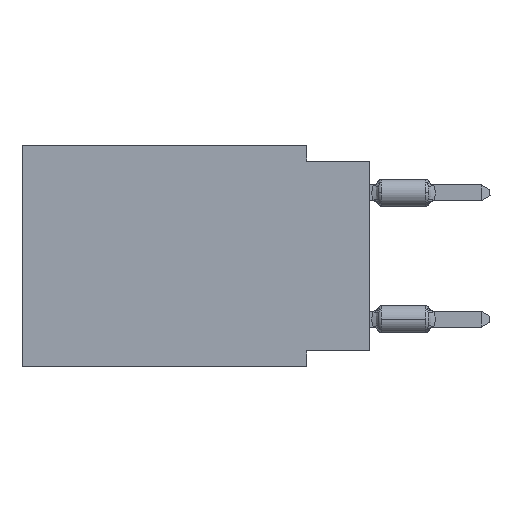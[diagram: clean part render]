
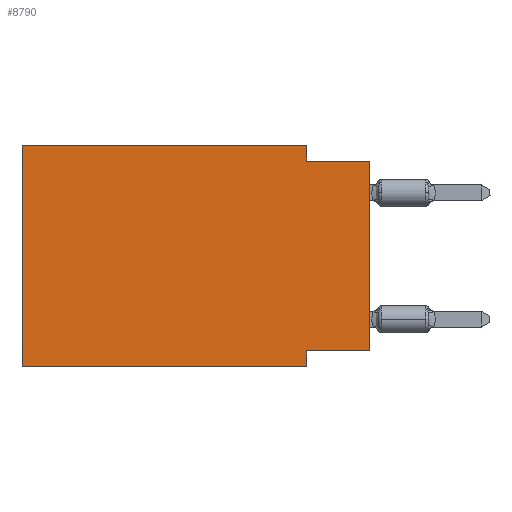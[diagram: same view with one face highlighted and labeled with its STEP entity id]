
A CAD part, left-side view. The second image highlights one B-rep face of the part: STEP entity #8790.
In plain terms, the highlighted planar face has unit normal (-1, 0, 0).
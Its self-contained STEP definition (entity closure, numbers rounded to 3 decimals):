
#327 = AXIS2_PLACEMENT_3D ( 'NONE', #10532, #20254, #37382 ) ;
#1716 = CARTESIAN_POINT ( 'NONE',  ( 0., 2.54, -8.89 ) ) ;
#2028 = VERTEX_POINT ( 'NONE', #53183 ) ;
#2197 = LINE ( 'NONE', #20183, #47291 ) ;
#2271 = PLANE ( 'NONE',  #327 ) ;
#3579 = CARTESIAN_POINT ( 'NONE',  ( 0., 13.97, 0. ) ) ;
#5478 = LINE ( 'NONE', #28453, #56012 ) ;
#7317 = CARTESIAN_POINT ( 'NONE',  ( 0., 2.54, 0. ) ) ;
#8790 = ADVANCED_FACE ( 'NONE', ( #19667 ), #2271, .F. ) ;
#9398 = VECTOR ( 'NONE', #21600, 1000. ) ;
#10532 = CARTESIAN_POINT ( 'NONE',  ( 0., 13.97, 0. ) ) ;
#11060 = DIRECTION ( 'NONE',  ( 0., -1., 0. ) ) ;
#11379 = DIRECTION ( 'NONE',  ( 0., 0., 1. ) ) ;
#12383 = VECTOR ( 'NONE', #16252, 1000. ) ;
#12592 = ORIENTED_EDGE ( 'NONE', *, *, #21545, .F. ) ;
#12681 = VECTOR ( 'NONE', #56651, 1000. ) ;
#12955 = VECTOR ( 'NONE', #26586, 1000. ) ;
#13992 = VERTEX_POINT ( 'NONE', #37721 ) ;
#14614 = VECTOR ( 'NONE', #56558, 1000. ) ;
#14849 = EDGE_CURVE ( 'NONE', #48085, #39375, #24808, .T. ) ;
#15495 = DIRECTION ( 'NONE',  ( 0., 0., -1. ) ) ;
#16252 = DIRECTION ( 'NONE',  ( 0., 0., 1. ) ) ;
#16602 = ORIENTED_EDGE ( 'NONE', *, *, #47740, .F. ) ;
#17611 = ORIENTED_EDGE ( 'NONE', *, *, #43153, .T. ) ;
#19488 = CARTESIAN_POINT ( 'NONE',  ( 0., 13.97, 0. ) ) ;
#19639 = CARTESIAN_POINT ( 'NONE',  ( 0., 0., 0. ) ) ;
#19667 = FACE_OUTER_BOUND ( 'NONE', #22935, .T. ) ;
#20183 = CARTESIAN_POINT ( 'NONE',  ( 0., 13.97, -8.89 ) ) ;
#20254 = DIRECTION ( 'NONE',  ( 1., 0., 0. ) ) ;
#20385 = CARTESIAN_POINT ( 'NONE',  ( 0., 0., -0.635 ) ) ;
#21545 = EDGE_CURVE ( 'NONE', #54140, #41581, #52586, .T. ) ;
#21600 = DIRECTION ( 'NONE',  ( 0., 1., 0. ) ) ;
#22935 = EDGE_LOOP ( 'NONE', ( #57510, #30529, #39712, #31897, #30223, #17611, #16602, #12592 ) ) ;
#24808 = LINE ( 'NONE', #20385, #12681 ) ;
#25574 = LINE ( 'NONE', #7317, #14614 ) ;
#25982 = LINE ( 'NONE', #3579, #12383 ) ;
#26586 = DIRECTION ( 'NONE',  ( 0., -1., 0. ) ) ;
#26988 = VERTEX_POINT ( 'NONE', #1716 ) ;
#28302 = VERTEX_POINT ( 'NONE', #19488 ) ;
#28453 = CARTESIAN_POINT ( 'NONE',  ( 0., 2.54, -8.89 ) ) ;
#30223 = ORIENTED_EDGE ( 'NONE', *, *, #42631, .F. ) ;
#30529 = ORIENTED_EDGE ( 'NONE', *, *, #14849, .F. ) ;
#31897 = ORIENTED_EDGE ( 'NONE', *, *, #52980, .F. ) ;
#33515 = CARTESIAN_POINT ( 'NONE',  ( 0., 0., -8.255 ) ) ;
#37382 = DIRECTION ( 'NONE',  ( 0., 0., -1. ) ) ;
#37721 = CARTESIAN_POINT ( 'NONE',  ( 0., 13.97, -8.89 ) ) ;
#39375 = VERTEX_POINT ( 'NONE', #53226 ) ;
#39712 = ORIENTED_EDGE ( 'NONE', *, *, #48692, .F. ) ;
#40180 = CARTESIAN_POINT ( 'NONE',  ( 0., 13.97, 0. ) ) ;
#41581 = VERTEX_POINT ( 'NONE', #50112 ) ;
#42631 = EDGE_CURVE ( 'NONE', #13992, #28302, #25982, .T. ) ;
#43153 = EDGE_CURVE ( 'NONE', #13992, #26988, #2197, .T. ) ;
#45451 = LINE ( 'NONE', #40180, #12955 ) ;
#47291 = VECTOR ( 'NONE', #11060, 1000. ) ;
#47740 = EDGE_CURVE ( 'NONE', #41581, #26988, #5478, .T. ) ;
#48085 = VERTEX_POINT ( 'NONE', #54078 ) ;
#48692 = EDGE_CURVE ( 'NONE', #2028, #48085, #25574, .T. ) ;
#50112 = CARTESIAN_POINT ( 'NONE',  ( 0., 2.54, -8.255 ) ) ;
#51420 = VECTOR ( 'NONE', #11379, 1000. ) ;
#51774 = LINE ( 'NONE', #19639, #51420 ) ;
#52586 = LINE ( 'NONE', #53161, #9398 ) ;
#52980 = EDGE_CURVE ( 'NONE', #28302, #2028, #45451, .T. ) ;
#53161 = CARTESIAN_POINT ( 'NONE',  ( 0., 0., -8.255 ) ) ;
#53183 = CARTESIAN_POINT ( 'NONE',  ( 0., 2.54, 0. ) ) ;
#53226 = CARTESIAN_POINT ( 'NONE',  ( 0., 0., -0.635 ) ) ;
#54078 = CARTESIAN_POINT ( 'NONE',  ( 0., 2.54, -0.635 ) ) ;
#54140 = VERTEX_POINT ( 'NONE', #33515 ) ;
#56012 = VECTOR ( 'NONE', #15495, 1000. ) ;
#56558 = DIRECTION ( 'NONE',  ( 0., 0., -1. ) ) ;
#56651 = DIRECTION ( 'NONE',  ( 0., -1., 0. ) ) ;
#57510 = ORIENTED_EDGE ( 'NONE', *, *, #57522, .T. ) ;
#57522 = EDGE_CURVE ( 'NONE', #54140, #39375, #51774, .T. ) ;
